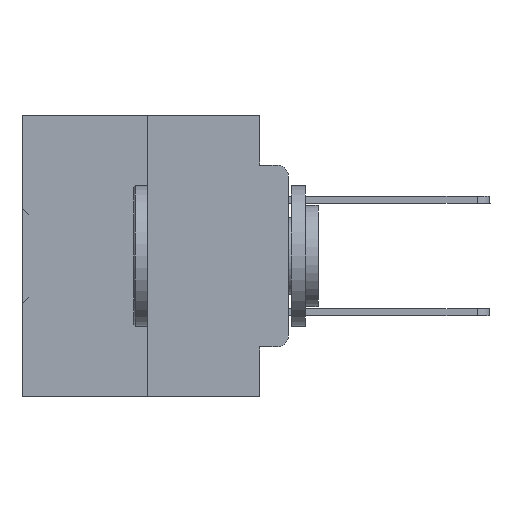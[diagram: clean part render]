
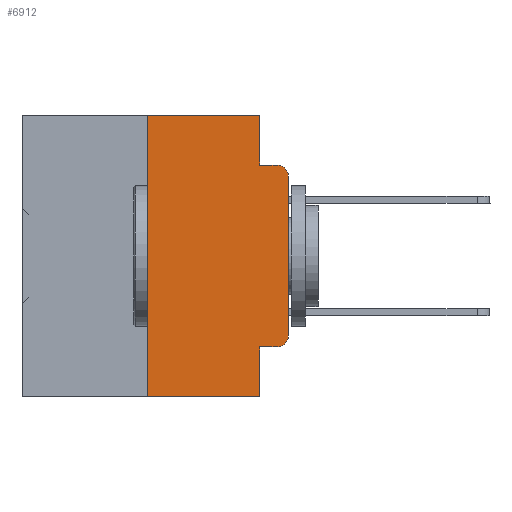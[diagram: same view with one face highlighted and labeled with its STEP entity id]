
A CAD part, left-side view. The second image highlights one B-rep face of the part: STEP entity #6912.
In plain terms, the highlighted planar face has unit normal (-1, 0, 0).
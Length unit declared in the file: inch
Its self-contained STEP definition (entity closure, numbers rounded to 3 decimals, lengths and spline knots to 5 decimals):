
#60 = EDGE_LOOP ( 'NONE', ( #38419, #4194, #7885, #23675, #24191, #8094, #20712, #27407, #13330, #39315 ) ) ;
#573 = EDGE_CURVE ( 'NONE', #8002, #38927, #32168, .T. ) ;
#801 = DIRECTION ( 'NONE',  ( -1., 0., 0. ) ) ;
#984 = VERTEX_POINT ( 'NONE', #5189 ) ;
#1243 = VERTEX_POINT ( 'NONE', #25432 ) ;
#1816 = CARTESIAN_POINT ( 'NONE',  ( 0., 0.473, 0. ) ) ;
#1942 = CARTESIAN_POINT ( 'NONE',  ( 0., 0.02, -0.4115 ) ) ;
#2321 = LINE ( 'NONE', #33660, #5170 ) ;
#2419 = DIRECTION ( 'NONE',  ( 0., 0., -1. ) ) ;
#3821 = AXIS2_PLACEMENT_3D ( 'NONE', #31142, #801, #6664 ) ;
#4194 = ORIENTED_EDGE ( 'NONE', *, *, #23328, .T. ) ;
#4212 = VECTOR ( 'NONE', #10603, 39.37008 ) ;
#4835 = LINE ( 'NONE', #1816, #20331 ) ;
#5155 = DIRECTION ( 'NONE',  ( 0., 0., -1. ) ) ;
#5170 = VECTOR ( 'NONE', #29830, 39.37008 ) ;
#5189 = CARTESIAN_POINT ( 'NONE',  ( 0., 0.02, -0.0885 ) ) ;
#5614 = VECTOR ( 'NONE', #35437, 39.37008 ) ;
#6341 = EDGE_CURVE ( 'NONE', #30858, #11550, #17248, .T. ) ;
#6507 = DIRECTION ( 'NONE',  ( -1., 0., 0. ) ) ;
#6664 = DIRECTION ( 'NONE',  ( 0., 0., -1. ) ) ;
#6912 = ADVANCED_FACE ( 'NONE', ( #11258 ), #39343, .F. ) ;
#7885 = ORIENTED_EDGE ( 'NONE', *, *, #31783, .F. ) ;
#8002 = VERTEX_POINT ( 'NONE', #10527 ) ;
#8094 = ORIENTED_EDGE ( 'NONE', *, *, #29925, .F. ) ;
#9437 = VECTOR ( 'NONE', #27128, 39.37008 ) ;
#10527 = CARTESIAN_POINT ( 'NONE',  ( 0., 0.051, 0. ) ) ;
#10603 = DIRECTION ( 'NONE',  ( 0., 0., -1. ) ) ;
#11028 = EDGE_CURVE ( 'NONE', #11550, #36750, #29113, .T. ) ;
#11258 = FACE_OUTER_BOUND ( 'NONE', #60, .T. ) ;
#11281 = VECTOR ( 'NONE', #38212, 39.37008 ) ;
#11550 = VERTEX_POINT ( 'NONE', #1942 ) ;
#12387 = DIRECTION ( 'NONE',  ( 0., 0., -1. ) ) ;
#13330 = ORIENTED_EDGE ( 'NONE', *, *, #6341, .T. ) ;
#13359 = VECTOR ( 'NONE', #2419, 39.37008 ) ;
#13657 = VECTOR ( 'NONE', #26527, 39.37008 ) ;
#14048 = VERTEX_POINT ( 'NONE', #24712 ) ;
#14369 = LINE ( 'NONE', #23677, #11281 ) ;
#14436 = CARTESIAN_POINT ( 'NONE',  ( 0., 0.25, 0. ) ) ;
#15945 = CARTESIAN_POINT ( 'NONE',  ( 0., 0., -0.3915 ) ) ;
#17210 = DIRECTION ( 'NONE',  ( 0., -1., 0. ) ) ;
#17248 = LINE ( 'NONE', #39253, #5614 ) ;
#18890 = EDGE_CURVE ( 'NONE', #36750, #1243, #14369, .T. ) ;
#18977 = EDGE_CURVE ( 'NONE', #21487, #8002, #4835, .T. ) ;
#20331 = VECTOR ( 'NONE', #17210, 39.37008 ) ;
#20617 = CIRCLE ( 'NONE', #3821, 0.02 ) ;
#20712 = ORIENTED_EDGE ( 'NONE', *, *, #37846, .T. ) ;
#21246 = CARTESIAN_POINT ( 'NONE',  ( 0., 0.051, 0. ) ) ;
#21487 = VERTEX_POINT ( 'NONE', #14436 ) ;
#22444 = CARTESIAN_POINT ( 'NONE',  ( 0., 0.051, -0.4115 ) ) ;
#23304 = CARTESIAN_POINT ( 'NONE',  ( 0., 0.473, -0.5 ) ) ;
#23328 = EDGE_CURVE ( 'NONE', #1243, #984, #20617, .T. ) ;
#23675 = ORIENTED_EDGE ( 'NONE', *, *, #573, .F. ) ;
#23677 = CARTESIAN_POINT ( 'NONE',  ( 0., 0., 0. ) ) ;
#24191 = ORIENTED_EDGE ( 'NONE', *, *, #18977, .F. ) ;
#24712 = CARTESIAN_POINT ( 'NONE',  ( 0., 0.051, -0.5 ) ) ;
#24800 = VERTEX_POINT ( 'NONE', #25754 ) ;
#25432 = CARTESIAN_POINT ( 'NONE',  ( 0., 0., -0.1085 ) ) ;
#25754 = CARTESIAN_POINT ( 'NONE',  ( 0., 0.25, -0.5 ) ) ;
#26527 = DIRECTION ( 'NONE',  ( 0., -1., 0. ) ) ;
#27128 = DIRECTION ( 'NONE',  ( 0., -1., 0. ) ) ;
#27407 = ORIENTED_EDGE ( 'NONE', *, *, #37327, .F. ) ;
#29113 = CIRCLE ( 'NONE', #33622, 0.02 ) ;
#29830 = DIRECTION ( 'NONE',  ( 0., 0., 1. ) ) ;
#29925 = EDGE_CURVE ( 'NONE', #24800, #21487, #2321, .T. ) ;
#30858 = VERTEX_POINT ( 'NONE', #22444 ) ;
#31010 = CARTESIAN_POINT ( 'NONE',  ( 0., 0.051, -0.0885 ) ) ;
#31142 = CARTESIAN_POINT ( 'NONE',  ( 0., 0.02, -0.1085 ) ) ;
#31783 = EDGE_CURVE ( 'NONE', #38927, #984, #38640, .T. ) ;
#32168 = LINE ( 'NONE', #21246, #13359 ) ;
#32479 = DIRECTION ( 'NONE',  ( 1., 0., 0. ) ) ;
#32819 = AXIS2_PLACEMENT_3D ( 'NONE', #38743, #32479, #5155 ) ;
#32983 = LINE ( 'NONE', #23304, #9437 ) ;
#33622 = AXIS2_PLACEMENT_3D ( 'NONE', #36854, #6507, #12387 ) ;
#33660 = CARTESIAN_POINT ( 'NONE',  ( 0., 0.25, 0. ) ) ;
#35074 = LINE ( 'NONE', #38497, #4212 ) ;
#35212 = CARTESIAN_POINT ( 'NONE',  ( 0., 0.051, -0.0885 ) ) ;
#35437 = DIRECTION ( 'NONE',  ( 0., -1., 0. ) ) ;
#36750 = VERTEX_POINT ( 'NONE', #15945 ) ;
#36854 = CARTESIAN_POINT ( 'NONE',  ( 0., 0.02, -0.3915 ) ) ;
#37327 = EDGE_CURVE ( 'NONE', #30858, #14048, #35074, .T. ) ;
#37846 = EDGE_CURVE ( 'NONE', #24800, #14048, #32983, .T. ) ;
#38212 = DIRECTION ( 'NONE',  ( 0., 0., 1. ) ) ;
#38419 = ORIENTED_EDGE ( 'NONE', *, *, #18890, .T. ) ;
#38497 = CARTESIAN_POINT ( 'NONE',  ( 0., 0.051, 0. ) ) ;
#38640 = LINE ( 'NONE', #35212, #13657 ) ;
#38743 = CARTESIAN_POINT ( 'NONE',  ( 0., 0.473, 0. ) ) ;
#38927 = VERTEX_POINT ( 'NONE', #31010 ) ;
#39253 = CARTESIAN_POINT ( 'NONE',  ( 0., 0.051, -0.4115 ) ) ;
#39315 = ORIENTED_EDGE ( 'NONE', *, *, #11028, .T. ) ;
#39343 = PLANE ( 'NONE',  #32819 ) ;
